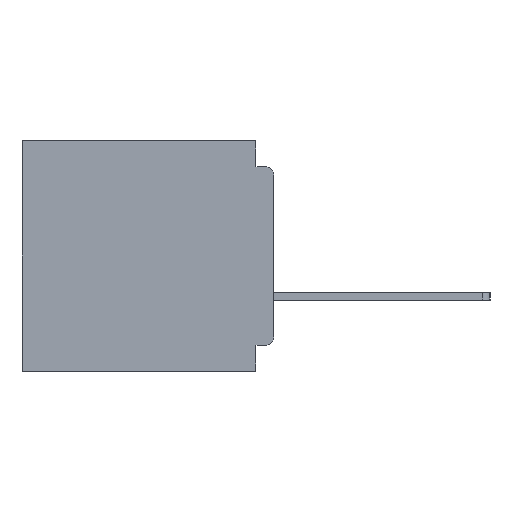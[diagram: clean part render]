
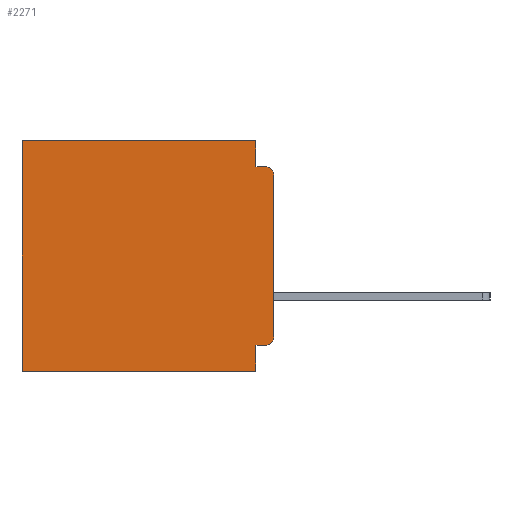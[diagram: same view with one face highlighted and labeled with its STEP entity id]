
A CAD part, left-side view. The second image highlights one B-rep face of the part: STEP entity #2271.
In plain terms, the highlighted planar face has unit normal (-1, 0, 0).
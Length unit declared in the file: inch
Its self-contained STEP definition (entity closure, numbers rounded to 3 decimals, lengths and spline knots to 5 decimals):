
#677 = CARTESIAN_POINT ( 'NONE',  ( 0.3, 0.015, -0.045 ) ) ;
#2271 = ADVANCED_FACE ( 'NONE', ( #21618 ), #42081, .F. ) ;
#2286 = AXIS2_PLACEMENT_3D ( 'NONE', #24533, #3204, #28097 ) ;
#2556 = DIRECTION ( 'NONE',  ( -1., 0., 0. ) ) ;
#2725 = EDGE_CURVE ( 'NONE', #8651, #18840, #12145, .T. ) ;
#2875 = ORIENTED_EDGE ( 'NONE', *, *, #31443, .T. ) ;
#3204 = DIRECTION ( 'NONE',  ( -1., 0., 0. ) ) ;
#3457 = EDGE_CURVE ( 'NONE', #25174, #5515, #15409, .T. ) ;
#3687 = CARTESIAN_POINT ( 'NONE',  ( 0.3, 0., 0. ) ) ;
#4282 = ORIENTED_EDGE ( 'NONE', *, *, #20256, .T. ) ;
#4735 = CARTESIAN_POINT ( 'NONE',  ( 0.3, 0., -0.4 ) ) ;
#5515 = VERTEX_POINT ( 'NONE', #13230 ) ;
#5563 = AXIS2_PLACEMENT_3D ( 'NONE', #4735, #26117, #18515 ) ;
#5784 = EDGE_CURVE ( 'NONE', #25733, #42299, #25161, .T. ) ;
#6077 = DIRECTION ( 'NONE',  ( 0., -1., 0. ) ) ;
#6774 = LINE ( 'NONE', #20248, #15155 ) ;
#7503 = VECTOR ( 'NONE', #32166, 39.37008 ) ;
#8651 = VERTEX_POINT ( 'NONE', #26538 ) ;
#10398 = EDGE_CURVE ( 'NONE', #18840, #25174, #20410, .T. ) ;
#10673 = EDGE_CURVE ( 'NONE', #45027, #29278, #35401, .T. ) ;
#10929 = CARTESIAN_POINT ( 'NONE',  ( 0.3, 0., -0.4 ) ) ;
#10957 = VECTOR ( 'NONE', #25927, 39.37008 ) ;
#11544 = LINE ( 'NONE', #10929, #28223 ) ;
#11545 = ORIENTED_EDGE ( 'NONE', *, *, #5784, .F. ) ;
#11556 = DIRECTION ( 'NONE',  ( 0., 1., 0. ) ) ;
#12027 = EDGE_CURVE ( 'NONE', #25733, #36343, #18116, .T. ) ;
#12145 = LINE ( 'NONE', #18202, #20469 ) ;
#12292 = CARTESIAN_POINT ( 'NONE',  ( 0.3, 0.437, 0. ) ) ;
#12588 = LINE ( 'NONE', #39747, #20904 ) ;
#12805 = ORIENTED_EDGE ( 'NONE', *, *, #10398, .F. ) ;
#13230 = CARTESIAN_POINT ( 'NONE',  ( 0.3, 0.437, -0.4 ) ) ;
#14289 = VERTEX_POINT ( 'NONE', #20659 ) ;
#14525 = DIRECTION ( 'NONE',  ( 0., 0., -1. ) ) ;
#14618 = VECTOR ( 'NONE', #36324, 39.37008 ) ;
#14963 = DIRECTION ( 'NONE',  ( 0., 0., -1. ) ) ;
#15155 = VECTOR ( 'NONE', #6077, 39.37008 ) ;
#15409 = LINE ( 'NONE', #27682, #33175 ) ;
#15715 = EDGE_CURVE ( 'NONE', #42299, #29278, #6774, .T. ) ;
#18116 = LINE ( 'NONE', #3687, #7503 ) ;
#18202 = CARTESIAN_POINT ( 'NONE',  ( 0.3, 0., -0.355 ) ) ;
#18515 = DIRECTION ( 'NONE',  ( 0., 0., -1. ) ) ;
#18840 = VERTEX_POINT ( 'NONE', #31703 ) ;
#19114 = ORIENTED_EDGE ( 'NONE', *, *, #2725, .F. ) ;
#20248 = CARTESIAN_POINT ( 'NONE',  ( 0.3, 0., -0.045 ) ) ;
#20256 = EDGE_CURVE ( 'NONE', #36343, #5515, #12588, .T. ) ;
#20410 = LINE ( 'NONE', #22342, #10957 ) ;
#20469 = VECTOR ( 'NONE', #11556, 39.37008 ) ;
#20659 = CARTESIAN_POINT ( 'NONE',  ( 0.3, 0., -0.34 ) ) ;
#20904 = VECTOR ( 'NONE', #14963, 39.37008 ) ;
#21618 = FACE_OUTER_BOUND ( 'NONE', #33145, .T. ) ;
#22167 = CIRCLE ( 'NONE', #2286, 0.015 ) ;
#22342 = CARTESIAN_POINT ( 'NONE',  ( 0.3, 0.031, -0.4 ) ) ;
#23903 = CARTESIAN_POINT ( 'NONE',  ( 0.3, 0.015, -0.06 ) ) ;
#24533 = CARTESIAN_POINT ( 'NONE',  ( 0.3, 0.015, -0.34 ) ) ;
#25161 = LINE ( 'NONE', #32751, #14618 ) ;
#25174 = VERTEX_POINT ( 'NONE', #28525 ) ;
#25733 = VERTEX_POINT ( 'NONE', #31760 ) ;
#25927 = DIRECTION ( 'NONE',  ( 0., 0., -1. ) ) ;
#26117 = DIRECTION ( 'NONE',  ( 1., 0., 0. ) ) ;
#26538 = CARTESIAN_POINT ( 'NONE',  ( 0.3, 0.015, -0.355 ) ) ;
#26737 = AXIS2_PLACEMENT_3D ( 'NONE', #23903, #2556, #27462 ) ;
#27462 = DIRECTION ( 'NONE',  ( 0., 0., -1. ) ) ;
#27682 = CARTESIAN_POINT ( 'NONE',  ( 0.3, 0., -0.4 ) ) ;
#28097 = DIRECTION ( 'NONE',  ( 0., 0., -1. ) ) ;
#28223 = VECTOR ( 'NONE', #14525, 39.37008 ) ;
#28525 = CARTESIAN_POINT ( 'NONE',  ( 0.3, 0.031, -0.4 ) ) ;
#29014 = ORIENTED_EDGE ( 'NONE', *, *, #10673, .T. ) ;
#29278 = VERTEX_POINT ( 'NONE', #677 ) ;
#29390 = DIRECTION ( 'NONE',  ( 0., 1., 0. ) ) ;
#29868 = ORIENTED_EDGE ( 'NONE', *, *, #15715, .F. ) ;
#30257 = CARTESIAN_POINT ( 'NONE',  ( 0.3, 0., -0.06 ) ) ;
#31443 = EDGE_CURVE ( 'NONE', #8651, #14289, #22167, .T. ) ;
#31703 = CARTESIAN_POINT ( 'NONE',  ( 0.3, 0.031, -0.355 ) ) ;
#31760 = CARTESIAN_POINT ( 'NONE',  ( 0.3, 0.031, 0. ) ) ;
#32166 = DIRECTION ( 'NONE',  ( 0., 1., 0. ) ) ;
#32751 = CARTESIAN_POINT ( 'NONE',  ( 0.3, 0.031, 0. ) ) ;
#32822 = EDGE_CURVE ( 'NONE', #45027, #14289, #11544, .T. ) ;
#33145 = EDGE_LOOP ( 'NONE', ( #39459, #29014, #29868, #11545, #38607, #4282, #36466, #12805, #19114, #2875 ) ) ;
#33175 = VECTOR ( 'NONE', #29390, 39.37008 ) ;
#35401 = CIRCLE ( 'NONE', #26737, 0.015 ) ;
#36324 = DIRECTION ( 'NONE',  ( 0., 0., -1. ) ) ;
#36343 = VERTEX_POINT ( 'NONE', #12292 ) ;
#36466 = ORIENTED_EDGE ( 'NONE', *, *, #3457, .F. ) ;
#38607 = ORIENTED_EDGE ( 'NONE', *, *, #12027, .T. ) ;
#39459 = ORIENTED_EDGE ( 'NONE', *, *, #32822, .F. ) ;
#39747 = CARTESIAN_POINT ( 'NONE',  ( 0.3, 0.437, -0.4 ) ) ;
#42081 = PLANE ( 'NONE',  #5563 ) ;
#42299 = VERTEX_POINT ( 'NONE', #43718 ) ;
#43718 = CARTESIAN_POINT ( 'NONE',  ( 0.3, 0.031, -0.045 ) ) ;
#45027 = VERTEX_POINT ( 'NONE', #30257 ) ;
